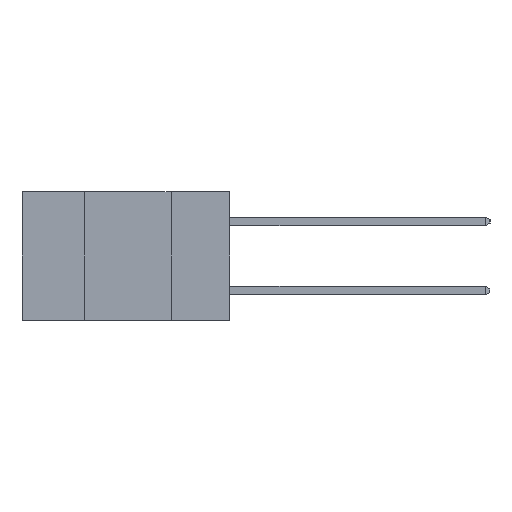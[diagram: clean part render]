
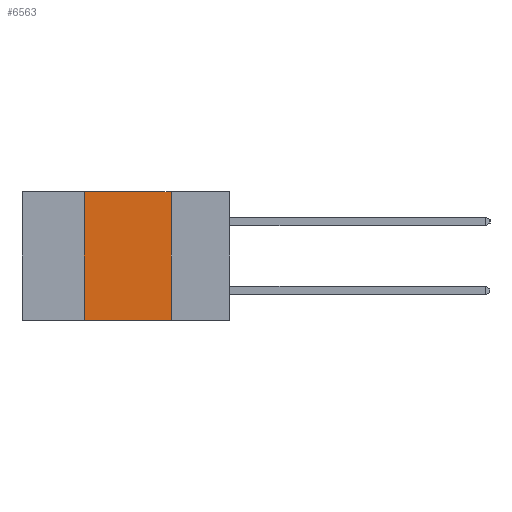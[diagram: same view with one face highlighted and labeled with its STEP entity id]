
A CAD part, left-side view. The second image highlights one B-rep face of the part: STEP entity #6563.
In plain terms, the highlighted planar face has unit normal (-1, 0, 0).
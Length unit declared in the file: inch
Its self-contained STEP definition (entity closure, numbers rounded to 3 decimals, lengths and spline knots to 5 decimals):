
#33 = ORIENTED_EDGE ( 'NONE', *, *, #7346, .F. ) ;
#685 = ORIENTED_EDGE ( 'NONE', *, *, #5586, .T. ) ;
#979 = CARTESIAN_POINT ( 'NONE',  ( 0., 0.17, 0. ) ) ;
#999 = ORIENTED_EDGE ( 'NONE', *, *, #12740, .F. ) ;
#1505 = AXIS2_PLACEMENT_3D ( 'NONE', #9801, #10980, #6508 ) ;
#2124 = DIRECTION ( 'NONE',  ( 0., 0., 1. ) ) ;
#2559 = LINE ( 'NONE', #12709, #12781 ) ;
#2988 = ORIENTED_EDGE ( 'NONE', *, *, #7160, .F. ) ;
#3179 = LINE ( 'NONE', #7242, #8447 ) ;
#3752 = VERTEX_POINT ( 'NONE', #5381 ) ;
#3951 = VERTEX_POINT ( 'NONE', #7145 ) ;
#4753 = VECTOR ( 'NONE', #11816, 39.37008 ) ;
#5381 = CARTESIAN_POINT ( 'NONE',  ( 0., 0.42, 0. ) ) ;
#5388 = VERTEX_POINT ( 'NONE', #12161 ) ;
#5586 = EDGE_CURVE ( 'NONE', #5388, #3951, #10399, .T. ) ;
#5707 = VERTEX_POINT ( 'NONE', #11289 ) ;
#5789 = DIRECTION ( 'NONE',  ( 0., -1., 0. ) ) ;
#6508 = DIRECTION ( 'NONE',  ( 0., 0., -1. ) ) ;
#6522 = CARTESIAN_POINT ( 'NONE',  ( 0., 0.6, -0.37 ) ) ;
#6563 = ADVANCED_FACE ( 'NONE', ( #6937 ), #11120, .F. ) ;
#6937 = FACE_OUTER_BOUND ( 'NONE', #9181, .T. ) ;
#7145 = CARTESIAN_POINT ( 'NONE',  ( 0., 0.17, -0.37 ) ) ;
#7160 = EDGE_CURVE ( 'NONE', #3752, #5707, #2559, .T. ) ;
#7242 = CARTESIAN_POINT ( 'NONE',  ( 0., 0.42, 0. ) ) ;
#7346 = EDGE_CURVE ( 'NONE', #5707, #3951, #10988, .T. ) ;
#8252 = VECTOR ( 'NONE', #10167, 39.37008 ) ;
#8447 = VECTOR ( 'NONE', #2124, 39.37008 ) ;
#9181 = EDGE_LOOP ( 'NONE', ( #33, #2988, #999, #685 ) ) ;
#9801 = CARTESIAN_POINT ( 'NONE',  ( 0., 0.6, 0. ) ) ;
#10167 = DIRECTION ( 'NONE',  ( 0., 0., -1. ) ) ;
#10399 = LINE ( 'NONE', #6522, #4753 ) ;
#10980 = DIRECTION ( 'NONE',  ( 1., 0., 0. ) ) ;
#10988 = LINE ( 'NONE', #979, #8252 ) ;
#11120 = PLANE ( 'NONE',  #1505 ) ;
#11289 = CARTESIAN_POINT ( 'NONE',  ( 0., 0.17, 0. ) ) ;
#11816 = DIRECTION ( 'NONE',  ( 0., -1., 0. ) ) ;
#12161 = CARTESIAN_POINT ( 'NONE',  ( 0., 0.42, -0.37 ) ) ;
#12709 = CARTESIAN_POINT ( 'NONE',  ( 0., 0.6, 0. ) ) ;
#12740 = EDGE_CURVE ( 'NONE', #5388, #3752, #3179, .T. ) ;
#12781 = VECTOR ( 'NONE', #5789, 39.37008 ) ;
